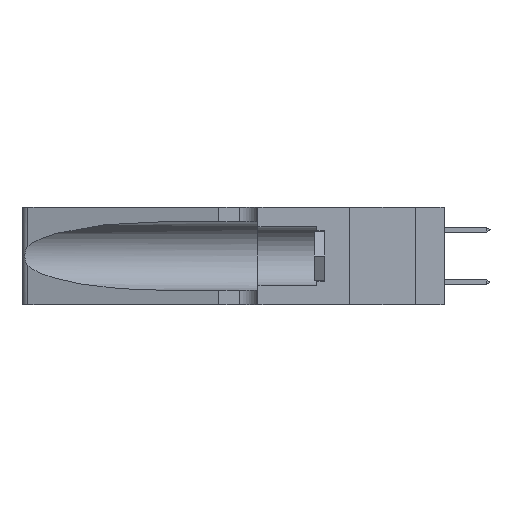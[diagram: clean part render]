
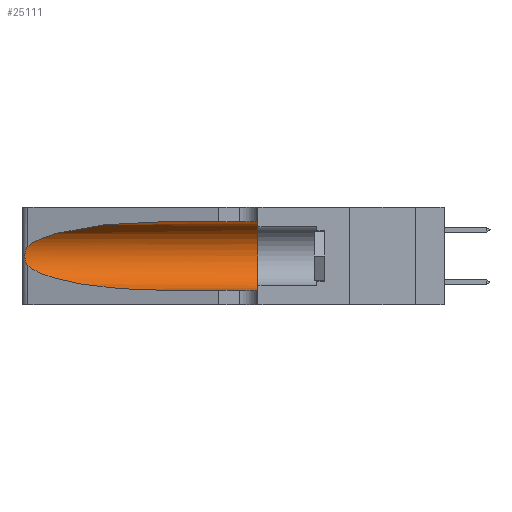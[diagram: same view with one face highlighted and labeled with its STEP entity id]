
A CAD part, left-side view. The second image highlights one B-rep face of the part: STEP entity #25111.
In plain terms, the highlighted cylindrical face has radius 3.308 mm (diameter 6.617 mm), a partial arc.
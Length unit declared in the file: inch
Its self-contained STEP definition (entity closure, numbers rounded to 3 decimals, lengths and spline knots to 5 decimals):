
#18 = CARTESIAN_POINT ( 'NONE',  ( 0.25487, 1.22718, 0.14631 ) ) ;
#490 = CARTESIAN_POINT ( 'NONE',  ( 0.1305, 0.72297, 0.05475 ) ) ;
#1598 = CARTESIAN_POINT ( 'NONE',  ( 0.1305, 1.61858, 0.185 ) ) ;
#2109 = CARTESIAN_POINT ( 'NONE',  ( 0.25639, 1.23184, 0.21858 ) ) ;
#2731 = VERTEX_POINT ( 'NONE', #15616 ) ;
#3414 = EDGE_CURVE ( 'NONE', #27402, #11564, #14358, .T. ) ;
#3710 = DIRECTION ( 'NONE',  ( 0., 0., 1. ) ) ;
#3745 = CIRCLE ( 'NONE', #15819, 0.13025 ) ;
#4004 = DIRECTION ( 'NONE',  ( 0., -1., 0. ) ) ;
#4211 = CARTESIAN_POINT ( 'NONE',  ( 0.25487, 1.22718, 0.22369 ) ) ;
#4802 = CARTESIAN_POINT ( 'NONE',  ( 0.1305, 0.72297, 0.31525 ) ) ;
#6455 = CARTESIAN_POINT ( 'NONE',  ( 0.25789, 1.23486, 0.15765 ) ) ;
#7052 = VECTOR ( 'NONE', #26578, 39.37008 ) ;
#7191 = AXIS2_PLACEMENT_3D ( 'NONE', #1598, #4004, #28809 ) ;
#7269 = VERTEX_POINT ( 'NONE', #23835 ) ;
#7282 = CARTESIAN_POINT ( 'NONE',  ( 0.25487, 1.22718, 0.22369 ) ) ;
#8150 = EDGE_CURVE ( 'NONE', #26892, #28055, #3745, .T. ) ;
#8326 = VECTOR ( 'NONE', #14702, 39.37008 ) ;
#8472 = ORIENTED_EDGE ( 'NONE', *, *, #8150, .F. ) ;
#8663 = CARTESIAN_POINT ( 'NONE',  ( 0.26018, 1.23835, 0.19895 ) ) ;
#8864 = CARTESIAN_POINT ( 'NONE',  ( 0.25487, 1.22718, 0.14631 ) ) ;
#9923 = LINE ( 'NONE', #28959, #7052 ) ;
#11065 = CARTESIAN_POINT ( 'NONE',  ( 0.25555, 1.22993, 0.14849 ) ) ;
#11170 = CARTESIAN_POINT ( 'NONE',  ( 0.25787, 1.23484, 0.2124 ) ) ;
#11564 = VERTEX_POINT ( 'NONE', #11569 ) ;
#11569 = CARTESIAN_POINT ( 'NONE',  ( 0.25487, 1.22718, 0.22369 ) ) ;
#11876 = CARTESIAN_POINT ( 'NONE',  ( 0.18966, 0.96281, 0.31525 ) ) ;
#12363 = CARTESIAN_POINT ( 'NONE',  ( 0.1305, 1.61858, 0.31525 ) ) ;
#13081 = CARTESIAN_POINT ( 'NONE',  ( 0.26075, 1.23896, 0.19203 ) ) ;
#13129 = ORIENTED_EDGE ( 'NONE', *, *, #23499, .T. ) ;
#13909 = CARTESIAN_POINT ( 'NONE',  ( 0.2373, 1.15595, 0.08982 ) ) ;
#14358 =( BOUNDED_CURVE ( )  B_SPLINE_CURVE ( 3, ( #4802, #11876, #16764, #7282 ),
 .UNSPECIFIED., .F., .F. ) 
 B_SPLINE_CURVE_WITH_KNOTS ( ( 4, 4 ),
 ( 1.5708, 2.84003 ),
 .UNSPECIFIED. ) 
 CURVE ( )  GEOMETRIC_REPRESENTATION_ITEM ( )  RATIONAL_B_SPLINE_CURVE ( ( 1., 0.87, 0.87, 1. ) ) 
 REPRESENTATION_ITEM ( '' )  );
#14702 = DIRECTION ( 'NONE',  ( 0., -1., 0. ) ) ;
#15102 = DIRECTION ( 'NONE',  ( 0., 1., 0. ) ) ;
#15603 = CARTESIAN_POINT ( 'NONE',  ( 0.25555, 1.22994, 0.2215 ) ) ;
#15616 = CARTESIAN_POINT ( 'NONE',  ( 0.1305, 0.72297, 0.05475 ) ) ;
#15695 = CARTESIAN_POINT ( 'NONE',  ( 0.26075, 1.23896, 0.178 ) ) ;
#15819 = AXIS2_PLACEMENT_3D ( 'NONE', #22158, #15102, #3710 ) ;
#16434 = CARTESIAN_POINT ( 'NONE',  ( 0.1305, 0.72297, 0.31525 ) ) ;
#16751 = ORIENTED_EDGE ( 'NONE', *, *, #23243, .F. ) ;
#16764 = CARTESIAN_POINT ( 'NONE',  ( 0.2373, 1.15595, 0.28018 ) ) ;
#17049 = CARTESIAN_POINT ( 'NONE',  ( 0.1305, 0.35, 0.31525 ) ) ;
#18514 = FACE_OUTER_BOUND ( 'NONE', #25864, .T. ) ;
#19032 = CARTESIAN_POINT ( 'NONE',  ( 0.18966, 0.96281, 0.05475 ) ) ;
#19945 = CARTESIAN_POINT ( 'NONE',  ( 0.26017, 1.23833, 0.17102 ) ) ;
#20305 = CYLINDRICAL_SURFACE ( 'NONE', #7191, 0.13025 ) ;
#20561 = EDGE_CURVE ( 'NONE', #2731, #28055, #9923, .T. ) ;
#22158 = CARTESIAN_POINT ( 'NONE',  ( 0.1305, 0.35, 0.185 ) ) ;
#22242 = B_SPLINE_CURVE_WITH_KNOTS ( 'NONE', 3,
 ( #4211, #15603, #2109, #11170, #26932, #8663, #13081, #15695, #19945, #24751, #6455, #22564, #11065, #8864 ),
 .UNSPECIFIED., .F., .F.,
 ( 4, 2, 2, 2, 2, 2, 4 ),
 ( 0., 0.00027, 0.00053, 0.00107, 0.0016, 0.00187, 0.00214 ),
 .UNSPECIFIED. ) ;
#22401 = ORIENTED_EDGE ( 'NONE', *, *, #29210, .T. ) ;
#22564 = CARTESIAN_POINT ( 'NONE',  ( 0.25639, 1.23186, 0.15144 ) ) ;
#22988 = LINE ( 'NONE', #12363, #8326 ) ;
#23243 = EDGE_CURVE ( 'NONE', #27402, #26892, #22988, .T. ) ;
#23499 = EDGE_CURVE ( 'NONE', #11564, #7269, #22242, .T. ) ;
#23835 = CARTESIAN_POINT ( 'NONE',  ( 0.25487, 1.22718, 0.14631 ) ) ;
#23883 = ORIENTED_EDGE ( 'NONE', *, *, #3414, .T. ) ;
#24751 = CARTESIAN_POINT ( 'NONE',  ( 0.25856, 1.23593, 0.16098 ) ) ;
#25111 = ADVANCED_FACE ( 'NONE', ( #18514 ), #20305, .F. ) ;
#25792 = CARTESIAN_POINT ( 'NONE',  ( 0.1305, 0.35, 0.05475 ) ) ;
#25864 = EDGE_LOOP ( 'NONE', ( #23883, #13129, #22401, #26188, #8472, #16751 ) ) ;
#26188 = ORIENTED_EDGE ( 'NONE', *, *, #20561, .T. ) ;
#26578 = DIRECTION ( 'NONE',  ( 0., -1., 0. ) ) ;
#26892 = VERTEX_POINT ( 'NONE', #17049 ) ;
#26932 = CARTESIAN_POINT ( 'NONE',  ( 0.25854, 1.2359, 0.20912 ) ) ;
#27160 =( BOUNDED_CURVE ( )  B_SPLINE_CURVE ( 3, ( #18, #13909, #19032, #490 ),
 .UNSPECIFIED., .F., .F. ) 
 B_SPLINE_CURVE_WITH_KNOTS ( ( 4, 4 ),
 ( 3.44316, 4.71239 ),
 .UNSPECIFIED. ) 
 CURVE ( )  GEOMETRIC_REPRESENTATION_ITEM ( )  RATIONAL_B_SPLINE_CURVE ( ( 1., 0.87, 0.87, 1. ) ) 
 REPRESENTATION_ITEM ( '' )  );
#27402 = VERTEX_POINT ( 'NONE', #16434 ) ;
#28055 = VERTEX_POINT ( 'NONE', #25792 ) ;
#28809 = DIRECTION ( 'NONE',  ( 0., 0., -1. ) ) ;
#28959 = CARTESIAN_POINT ( 'NONE',  ( 0.1305, 1.61858, 0.05475 ) ) ;
#29210 = EDGE_CURVE ( 'NONE', #7269, #2731, #27160, .T. ) ;
